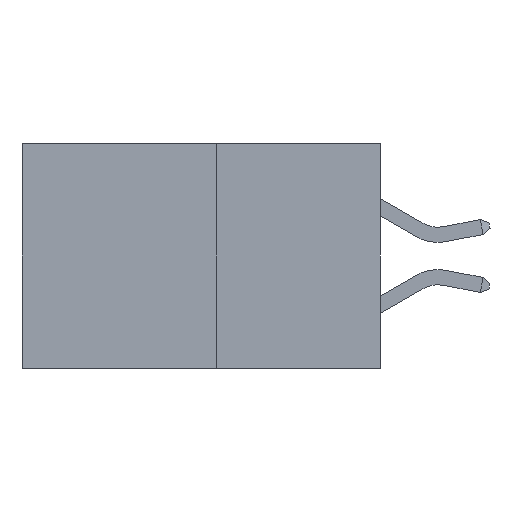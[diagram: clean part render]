
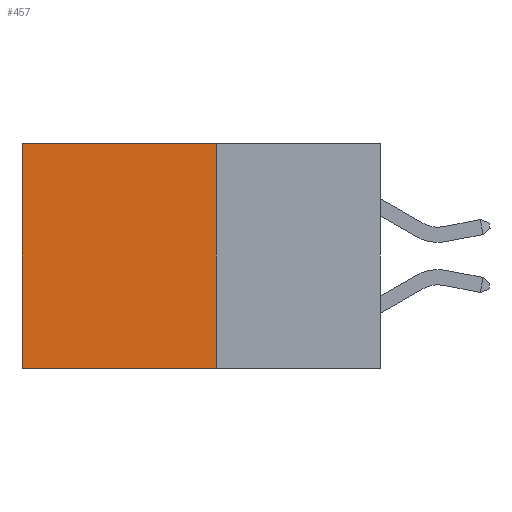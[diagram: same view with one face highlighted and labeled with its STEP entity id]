
A CAD part, left-side view. The second image highlights one B-rep face of the part: STEP entity #457.
In plain terms, the highlighted planar face has unit normal (-1, 0, 0).
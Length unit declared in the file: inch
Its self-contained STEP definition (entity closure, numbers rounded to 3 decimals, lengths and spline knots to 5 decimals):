
#7 = VECTOR ( 'NONE', #760, 39.37008 ) ;
#80 = EDGE_CURVE ( 'NONE', #7012, #9777, #2389, .T. ) ;
#428 = DIRECTION ( 'NONE',  ( 0., 0., -1. ) ) ;
#457 = ADVANCED_FACE ( 'NONE', ( #10977 ), #3739, .F. ) ;
#760 = DIRECTION ( 'NONE',  ( 0., 0., -1. ) ) ;
#1775 = CARTESIAN_POINT ( 'NONE',  ( 0.277, 0.27, -0.37 ) ) ;
#2222 = CARTESIAN_POINT ( 'NONE',  ( 0.277, 0.27, 0. ) ) ;
#2389 = LINE ( 'NONE', #7543, #7 ) ;
#2475 = EDGE_LOOP ( 'NONE', ( #3030, #3137, #4673, #6260 ) ) ;
#3030 = ORIENTED_EDGE ( 'NONE', *, *, #80, .T. ) ;
#3137 = ORIENTED_EDGE ( 'NONE', *, *, #7820, .F. ) ;
#3428 = VECTOR ( 'NONE', #10269, 39.37008 ) ;
#3739 = PLANE ( 'NONE',  #5930 ) ;
#4032 = VECTOR ( 'NONE', #6507, 39.37008 ) ;
#4457 = LINE ( 'NONE', #8348, #4924 ) ;
#4673 = ORIENTED_EDGE ( 'NONE', *, *, #11151, .F. ) ;
#4765 = CARTESIAN_POINT ( 'NONE',  ( 0.277, 0.27, 0. ) ) ;
#4832 = DIRECTION ( 'NONE',  ( 0., 0., -1. ) ) ;
#4924 = VECTOR ( 'NONE', #428, 39.37008 ) ;
#5118 = CARTESIAN_POINT ( 'NONE',  ( 0.277, 0.59, -0.37 ) ) ;
#5603 = CARTESIAN_POINT ( 'NONE',  ( 0.277, 0.27, -0.37 ) ) ;
#5905 = LINE ( 'NONE', #2222, #4032 ) ;
#5930 = AXIS2_PLACEMENT_3D ( 'NONE', #6995, #8675, #4832 ) ;
#6260 = ORIENTED_EDGE ( 'NONE', *, *, #6265, .T. ) ;
#6265 = EDGE_CURVE ( 'NONE', #7046, #7012, #5905, .T. ) ;
#6507 = DIRECTION ( 'NONE',  ( 0., 1., 0. ) ) ;
#6995 = CARTESIAN_POINT ( 'NONE',  ( 0.277, 0.27, -0.37 ) ) ;
#7012 = VERTEX_POINT ( 'NONE', #11179 ) ;
#7046 = VERTEX_POINT ( 'NONE', #4765 ) ;
#7092 = VERTEX_POINT ( 'NONE', #5603 ) ;
#7543 = CARTESIAN_POINT ( 'NONE',  ( 0.277, 0.59, -0.37 ) ) ;
#7820 = EDGE_CURVE ( 'NONE', #7092, #9777, #10002, .T. ) ;
#8348 = CARTESIAN_POINT ( 'NONE',  ( 0.277, 0.27, -0.37 ) ) ;
#8675 = DIRECTION ( 'NONE',  ( 1., 0., 0. ) ) ;
#9777 = VERTEX_POINT ( 'NONE', #5118 ) ;
#10002 = LINE ( 'NONE', #1775, #3428 ) ;
#10269 = DIRECTION ( 'NONE',  ( 0., 1., 0. ) ) ;
#10977 = FACE_OUTER_BOUND ( 'NONE', #2475, .T. ) ;
#11151 = EDGE_CURVE ( 'NONE', #7046, #7092, #4457, .T. ) ;
#11179 = CARTESIAN_POINT ( 'NONE',  ( 0.277, 0.59, 0. ) ) ;
